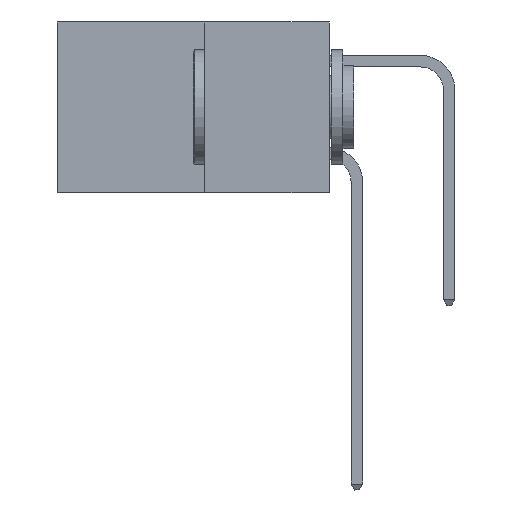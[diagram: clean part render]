
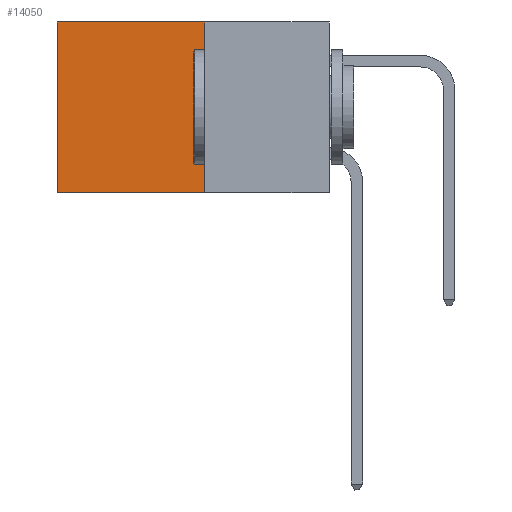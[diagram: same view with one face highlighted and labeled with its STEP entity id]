
A CAD part, left-side view. The second image highlights one B-rep face of the part: STEP entity #14050.
In plain terms, the highlighted planar face has unit normal (-1, 0, 0).
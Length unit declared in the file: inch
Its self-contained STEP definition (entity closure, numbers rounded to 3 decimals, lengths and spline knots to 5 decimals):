
#67 = LINE ( 'NONE', #9755, #12702 ) ;
#1616 = DIRECTION ( 'NONE',  ( 0., 0., -1. ) ) ;
#2066 = CARTESIAN_POINT ( 'NONE',  ( 0.277, 0.59, -0.37 ) ) ;
#2372 = VERTEX_POINT ( 'NONE', #8545 ) ;
#3022 = DIRECTION ( 'NONE',  ( 0., 1., 0. ) ) ;
#4603 = LINE ( 'NONE', #7318, #15821 ) ;
#4808 = AXIS2_PLACEMENT_3D ( 'NONE', #20644, #9471, #25060 ) ;
#7227 = PLANE ( 'NONE',  #4808 ) ;
#7318 = CARTESIAN_POINT ( 'NONE',  ( 0.277, 0.27, -0.37 ) ) ;
#8545 = CARTESIAN_POINT ( 'NONE',  ( 0.277, 0.59, 0. ) ) ;
#9471 = DIRECTION ( 'NONE',  ( 1., 0., 0. ) ) ;
#9755 = CARTESIAN_POINT ( 'NONE',  ( 0.277, 0.27, 0. ) ) ;
#10060 = VERTEX_POINT ( 'NONE', #2066 ) ;
#10084 = ORIENTED_EDGE ( 'NONE', *, *, #17388, .T. ) ;
#10925 = EDGE_CURVE ( 'NONE', #19969, #10060, #4603, .T. ) ;
#11083 = VECTOR ( 'NONE', #1616, 39.37008 ) ;
#12702 = VECTOR ( 'NONE', #3022, 39.37008 ) ;
#13805 = EDGE_CURVE ( 'NONE', #2372, #10060, #21902, .T. ) ;
#13947 = ORIENTED_EDGE ( 'NONE', *, *, #13805, .T. ) ;
#14050 = ADVANCED_FACE ( 'NONE', ( #27410 ), #7227, .F. ) ;
#15821 = VECTOR ( 'NONE', #22952, 39.37008 ) ;
#16038 = VECTOR ( 'NONE', #17641, 39.37008 ) ;
#17388 = EDGE_CURVE ( 'NONE', #27446, #2372, #67, .T. ) ;
#17641 = DIRECTION ( 'NONE',  ( 0., 0., -1. ) ) ;
#18862 = ORIENTED_EDGE ( 'NONE', *, *, #20557, .F. ) ;
#19343 = ORIENTED_EDGE ( 'NONE', *, *, #10925, .F. ) ;
#19671 = CARTESIAN_POINT ( 'NONE',  ( 0.277, 0.27, -0.37 ) ) ;
#19724 = EDGE_LOOP ( 'NONE', ( #13947, #19343, #18862, #10084 ) ) ;
#19969 = VERTEX_POINT ( 'NONE', #19671 ) ;
#20557 = EDGE_CURVE ( 'NONE', #27446, #19969, #23659, .T. ) ;
#20644 = CARTESIAN_POINT ( 'NONE',  ( 0.277, 0.27, -0.37 ) ) ;
#21902 = LINE ( 'NONE', #24215, #16038 ) ;
#22952 = DIRECTION ( 'NONE',  ( 0., 1., 0. ) ) ;
#23659 = LINE ( 'NONE', #28285, #11083 ) ;
#24215 = CARTESIAN_POINT ( 'NONE',  ( 0.277, 0.59, -0.37 ) ) ;
#25060 = DIRECTION ( 'NONE',  ( 0., 0., -1. ) ) ;
#27410 = FACE_OUTER_BOUND ( 'NONE', #19724, .T. ) ;
#27446 = VERTEX_POINT ( 'NONE', #28092 ) ;
#28092 = CARTESIAN_POINT ( 'NONE',  ( 0.277, 0.27, 0. ) ) ;
#28285 = CARTESIAN_POINT ( 'NONE',  ( 0.277, 0.27, -0.37 ) ) ;
